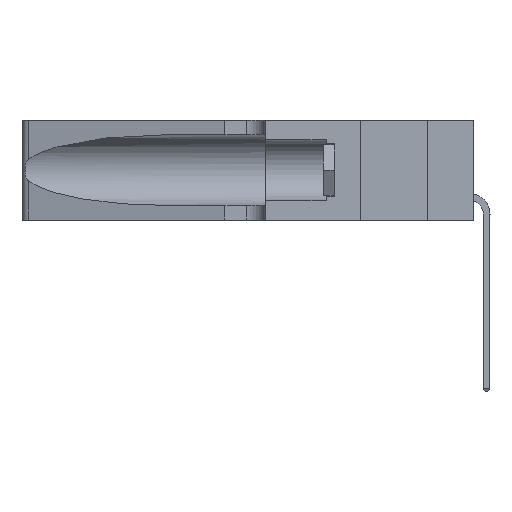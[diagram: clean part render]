
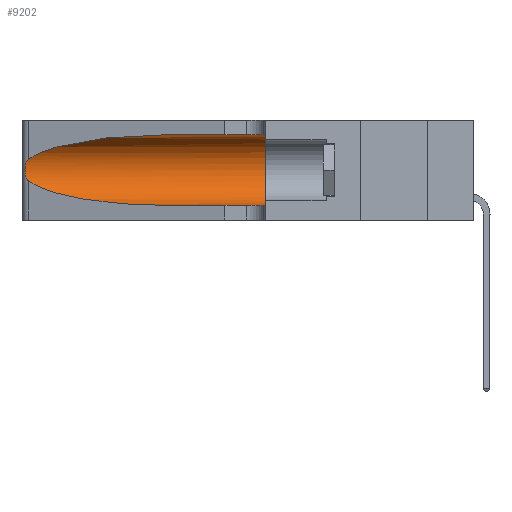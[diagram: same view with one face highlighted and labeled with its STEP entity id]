
A CAD part, left-side view. The second image highlights one B-rep face of the part: STEP entity #9202.
In plain terms, the highlighted cylindrical face has radius 3.308 mm (diameter 6.617 mm), a partial arc.
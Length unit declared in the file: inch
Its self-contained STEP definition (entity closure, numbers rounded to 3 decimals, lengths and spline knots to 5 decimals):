
#742 =( BOUNDED_CURVE ( )  B_SPLINE_CURVE ( 3, ( #41763, #6045, #9497, #28639 ),
 .UNSPECIFIED., .F., .F. ) 
 B_SPLINE_CURVE_WITH_KNOTS ( ( 4, 4 ),
 ( 3.44316, 4.71239 ),
 .UNSPECIFIED. ) 
 CURVE ( )  GEOMETRIC_REPRESENTATION_ITEM ( )  RATIONAL_B_SPLINE_CURVE ( ( 1., 0.87, 0.87, 1. ) ) 
 REPRESENTATION_ITEM ( '' )  );
#1232 = ORIENTED_EDGE ( 'NONE', *, *, #30974, .F. ) ;
#1297 = CARTESIAN_POINT ( 'NONE',  ( 0.1305, 0.35, 0.05475 ) ) ;
#2035 = CARTESIAN_POINT ( 'NONE',  ( 0.25555, 1.22993, 0.14849 ) ) ;
#2608 = CARTESIAN_POINT ( 'NONE',  ( 0.18966, 0.96281, 0.31525 ) ) ;
#3111 = VERTEX_POINT ( 'NONE', #16003 ) ;
#3861 = CARTESIAN_POINT ( 'NONE',  ( 0.1305, 1.61858, 0.05475 ) ) ;
#4057 = AXIS2_PLACEMENT_3D ( 'NONE', #9799, #6769, #39081 ) ;
#4129 = CARTESIAN_POINT ( 'NONE',  ( 0.1305, 0.35, 0.31525 ) ) ;
#4361 = VERTEX_POINT ( 'NONE', #15995 ) ;
#4963 = EDGE_CURVE ( 'NONE', #3111, #17200, #22397, .T. ) ;
#5644 = CARTESIAN_POINT ( 'NONE',  ( 0.25555, 1.22994, 0.2215 ) ) ;
#6032 = CYLINDRICAL_SURFACE ( 'NONE', #39703, 0.13025 ) ;
#6045 = CARTESIAN_POINT ( 'NONE',  ( 0.2373, 1.15595, 0.08982 ) ) ;
#6268 = DIRECTION ( 'NONE',  ( 0., 0., -1. ) ) ;
#6767 = EDGE_LOOP ( 'NONE', ( #36392, #30467, #16198, #7591, #19764, #1232 ) ) ;
#6769 = DIRECTION ( 'NONE',  ( 0., 1., 0. ) ) ;
#7591 = ORIENTED_EDGE ( 'NONE', *, *, #18148, .T. ) ;
#8954 = CARTESIAN_POINT ( 'NONE',  ( 0.25787, 1.23484, 0.2124 ) ) ;
#9025 = CARTESIAN_POINT ( 'NONE',  ( 0.1305, 1.61858, 0.185 ) ) ;
#9202 = ADVANCED_FACE ( 'NONE', ( #31912 ), #6032, .F. ) ;
#9497 = CARTESIAN_POINT ( 'NONE',  ( 0.18966, 0.96281, 0.05475 ) ) ;
#9799 = CARTESIAN_POINT ( 'NONE',  ( 0.1305, 0.35, 0.185 ) ) ;
#10728 = DIRECTION ( 'NONE',  ( 0., -1., 0. ) ) ;
#11043 = VERTEX_POINT ( 'NONE', #4129 ) ;
#11313 = CARTESIAN_POINT ( 'NONE',  ( 0.1305, 0.72297, 0.05475 ) ) ;
#12790 = CARTESIAN_POINT ( 'NONE',  ( 0.26075, 1.23896, 0.19203 ) ) ;
#15995 = CARTESIAN_POINT ( 'NONE',  ( 0.1305, 0.72297, 0.31525 ) ) ;
#16003 = CARTESIAN_POINT ( 'NONE',  ( 0.25487, 1.22718, 0.22369 ) ) ;
#16198 = ORIENTED_EDGE ( 'NONE', *, *, #28480, .T. ) ;
#17200 = VERTEX_POINT ( 'NONE', #36350 ) ;
#18013 = CARTESIAN_POINT ( 'NONE',  ( 0.25789, 1.23486, 0.15765 ) ) ;
#18148 = EDGE_CURVE ( 'NONE', #18359, #20024, #36473, .T. ) ;
#18153 = CARTESIAN_POINT ( 'NONE',  ( 0.26017, 1.23833, 0.17102 ) ) ;
#18359 = VERTEX_POINT ( 'NONE', #11313 ) ;
#19764 = ORIENTED_EDGE ( 'NONE', *, *, #36429, .F. ) ;
#20024 = VERTEX_POINT ( 'NONE', #1297 ) ;
#21263 = CARTESIAN_POINT ( 'NONE',  ( 0.25639, 1.23186, 0.15144 ) ) ;
#21825 = CARTESIAN_POINT ( 'NONE',  ( 0.26075, 1.23896, 0.178 ) ) ;
#22363 = DIRECTION ( 'NONE',  ( 0., -1., 0. ) ) ;
#22397 = B_SPLINE_CURVE_WITH_KNOTS ( 'NONE', 3,
 ( #38675, #5644, #28379, #8954, #31588, #38098, #12790, #21825, #18153, #34123, #18013, #21263, #2035, #24520 ),
 .UNSPECIFIED., .F., .F.,
 ( 4, 2, 2, 2, 2, 2, 4 ),
 ( 0., 0.00027, 0.00053, 0.00107, 0.0016, 0.00187, 0.00214 ),
 .UNSPECIFIED. ) ;
#23642 = CIRCLE ( 'NONE', #4057, 0.13025 ) ;
#24520 = CARTESIAN_POINT ( 'NONE',  ( 0.25487, 1.22718, 0.14631 ) ) ;
#28379 = CARTESIAN_POINT ( 'NONE',  ( 0.25639, 1.23184, 0.21858 ) ) ;
#28480 = EDGE_CURVE ( 'NONE', #17200, #18359, #742, .T. ) ;
#28639 = CARTESIAN_POINT ( 'NONE',  ( 0.1305, 0.72297, 0.05475 ) ) ;
#29891 = LINE ( 'NONE', #41105, #39454 ) ;
#30467 = ORIENTED_EDGE ( 'NONE', *, *, #4963, .T. ) ;
#30974 = EDGE_CURVE ( 'NONE', #4361, #11043, #29891, .T. ) ;
#31588 = CARTESIAN_POINT ( 'NONE',  ( 0.25854, 1.2359, 0.20912 ) ) ;
#31912 = FACE_OUTER_BOUND ( 'NONE', #6767, .T. ) ;
#32649 = CARTESIAN_POINT ( 'NONE',  ( 0.25487, 1.22718, 0.22369 ) ) ;
#32945 = VECTOR ( 'NONE', #10728, 39.37008 ) ;
#34123 = CARTESIAN_POINT ( 'NONE',  ( 0.25856, 1.23593, 0.16098 ) ) ;
#35779 = CARTESIAN_POINT ( 'NONE',  ( 0.2373, 1.15595, 0.28018 ) ) ;
#36350 = CARTESIAN_POINT ( 'NONE',  ( 0.25487, 1.22718, 0.14631 ) ) ;
#36392 = ORIENTED_EDGE ( 'NONE', *, *, #40176, .T. ) ;
#36429 = EDGE_CURVE ( 'NONE', #11043, #20024, #23642, .T. ) ;
#36473 = LINE ( 'NONE', #3861, #32945 ) ;
#37970 = DIRECTION ( 'NONE',  ( 0., -1., 0. ) ) ;
#38098 = CARTESIAN_POINT ( 'NONE',  ( 0.26018, 1.23835, 0.19895 ) ) ;
#38675 = CARTESIAN_POINT ( 'NONE',  ( 0.25487, 1.22718, 0.22369 ) ) ;
#39081 = DIRECTION ( 'NONE',  ( 0., 0., 1. ) ) ;
#39235 =( BOUNDED_CURVE ( )  B_SPLINE_CURVE ( 3, ( #41038, #2608, #35779, #32649 ),
 .UNSPECIFIED., .F., .F. ) 
 B_SPLINE_CURVE_WITH_KNOTS ( ( 4, 4 ),
 ( 1.5708, 2.84003 ),
 .UNSPECIFIED. ) 
 CURVE ( )  GEOMETRIC_REPRESENTATION_ITEM ( )  RATIONAL_B_SPLINE_CURVE ( ( 1., 0.87, 0.87, 1. ) ) 
 REPRESENTATION_ITEM ( '' )  );
#39454 = VECTOR ( 'NONE', #37970, 39.37008 ) ;
#39703 = AXIS2_PLACEMENT_3D ( 'NONE', #9025, #22363, #6268 ) ;
#40176 = EDGE_CURVE ( 'NONE', #4361, #3111, #39235, .T. ) ;
#41038 = CARTESIAN_POINT ( 'NONE',  ( 0.1305, 0.72297, 0.31525 ) ) ;
#41105 = CARTESIAN_POINT ( 'NONE',  ( 0.1305, 1.61858, 0.31525 ) ) ;
#41763 = CARTESIAN_POINT ( 'NONE',  ( 0.25487, 1.22718, 0.14631 ) ) ;
